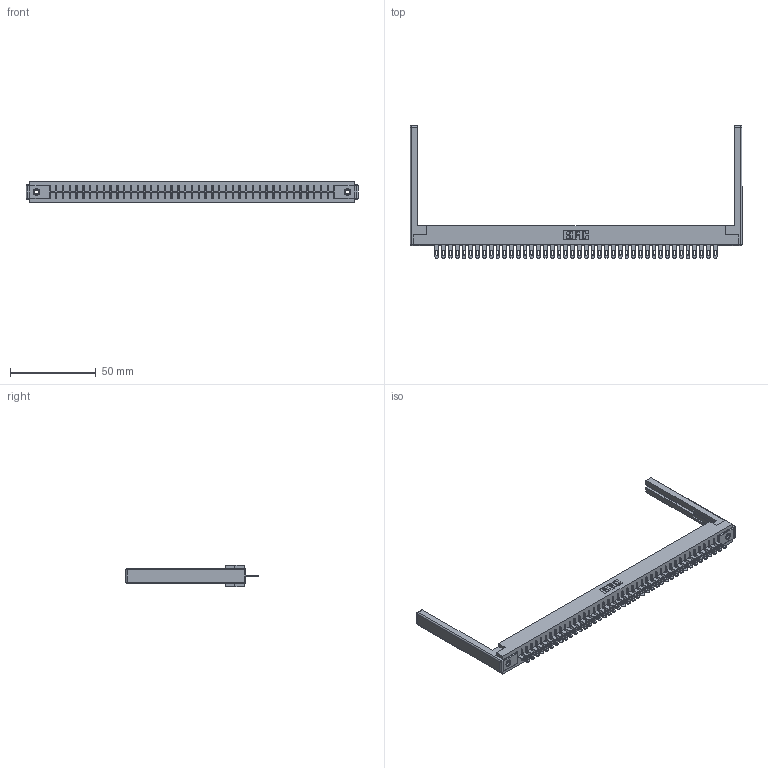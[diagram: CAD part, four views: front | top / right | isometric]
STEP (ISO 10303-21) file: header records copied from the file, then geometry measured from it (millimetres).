
FILE_DESCRIPTION (( 'STEP AP203' ), '1' );
FILE_NAME ('316-042-400-168.STEP', '2020-09-23T07:28:35', ( '' ), ( '' ), 'SwSTEP 2.0', 'SolidWorks 2020', '' );
FILE_SCHEMA (( 'CONFIG_CONTROL_DESIGN' ));
Length unit declared in the file: inch
Products named in the file (5): 316-042-400-168; 306 Part_.156 Dia; 306-290-001_100; 307-220-068; 345-250-001_345-250-001-102
Assembly tree (47 placements, depth 2):
  316-042-400-168
    306 Part_.156 Dia
    306-290-001_100  x42
    345-250-001_345-250-001-102  x2
    307-220-068  x2
Bounding box: 193.85 x 77.17 x 12.7 mm (x, y, z)
Volume: 25943.1 mm3; surface area: 26937.6 mm2
Topology: 47 solids, 47 shells, 3462 faces, 9736 edges, 6244 vertices
Faces by surface type: plane 2256, cylinder 1014, sphere 176, cone 12, torus 4
Entity records: 42090 total; most frequent: CARTESIAN_POINT 7034, ORIENTED_EDGE 6966, DIRECTION 6949, EDGE_CURVE 3483, LINE 2719, VECTOR 2719, VERTEX_POINT 2200, AXIS2_PLACEMENT_3D 2115
